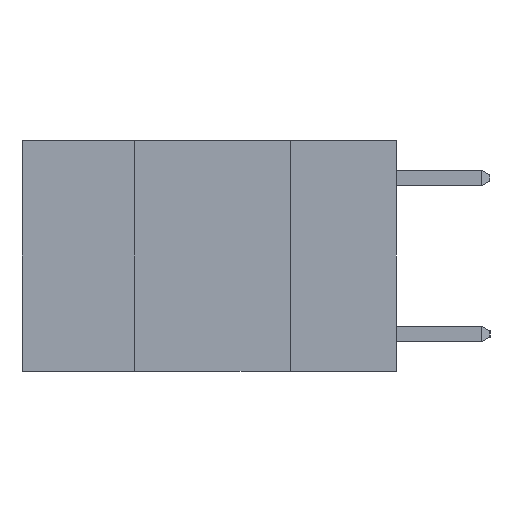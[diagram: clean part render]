
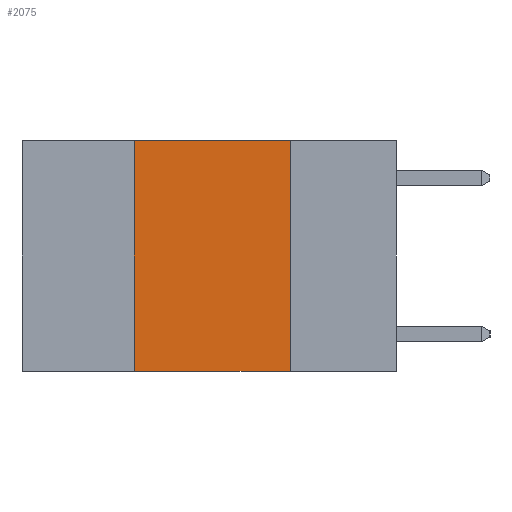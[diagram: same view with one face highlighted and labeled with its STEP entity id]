
A CAD part, left-side view. The second image highlights one B-rep face of the part: STEP entity #2075.
In plain terms, the highlighted planar face has unit normal (-1, 0, 0).
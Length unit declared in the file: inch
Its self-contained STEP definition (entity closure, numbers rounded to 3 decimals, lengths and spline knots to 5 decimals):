
#252 = CARTESIAN_POINT ( 'NONE',  ( 0., 0.6, -0.37 ) ) ;
#378 = EDGE_LOOP ( 'NONE', ( #4096, #4317, #6116, #4519 ) ) ;
#1094 = VECTOR ( 'NONE', #1281, 39.37008 ) ;
#1276 = CARTESIAN_POINT ( 'NONE',  ( 0., 0.42, 0. ) ) ;
#1281 = DIRECTION ( 'NONE',  ( 0., 0., -1. ) ) ;
#1657 = CARTESIAN_POINT ( 'NONE',  ( 0., 0.17, 0. ) ) ;
#2075 = ADVANCED_FACE ( 'NONE', ( #7980 ), #2799, .F. ) ;
#2078 = VECTOR ( 'NONE', #2474, 39.37008 ) ;
#2134 = CARTESIAN_POINT ( 'NONE',  ( 0., 0.17, 0. ) ) ;
#2190 = CARTESIAN_POINT ( 'NONE',  ( 0., 0.6, 0. ) ) ;
#2298 = EDGE_CURVE ( 'NONE', #8697, #3487, #2957, .T. ) ;
#2377 = EDGE_CURVE ( 'NONE', #8697, #4282, #5681, .T. ) ;
#2474 = DIRECTION ( 'NONE',  ( 0., -1., 0. ) ) ;
#2799 = PLANE ( 'NONE',  #4095 ) ;
#2909 = DIRECTION ( 'NONE',  ( 1., 0., 0. ) ) ;
#2939 = LINE ( 'NONE', #1657, #1094 ) ;
#2957 = LINE ( 'NONE', #1276, #8081 ) ;
#2985 = VECTOR ( 'NONE', #7218, 39.37008 ) ;
#3204 = VERTEX_POINT ( 'NONE', #2134 ) ;
#3212 = EDGE_CURVE ( 'NONE', #3204, #4282, #2939, .T. ) ;
#3487 = VERTEX_POINT ( 'NONE', #5888 ) ;
#4095 = AXIS2_PLACEMENT_3D ( 'NONE', #2190, #2909, #4097 ) ;
#4096 = ORIENTED_EDGE ( 'NONE', *, *, #3212, .F. ) ;
#4097 = DIRECTION ( 'NONE',  ( 0., 0., -1. ) ) ;
#4282 = VERTEX_POINT ( 'NONE', #7170 ) ;
#4317 = ORIENTED_EDGE ( 'NONE', *, *, #8198, .F. ) ;
#4519 = ORIENTED_EDGE ( 'NONE', *, *, #2377, .T. ) ;
#5395 = DIRECTION ( 'NONE',  ( 0., 0., 1. ) ) ;
#5681 = LINE ( 'NONE', #252, #2078 ) ;
#5888 = CARTESIAN_POINT ( 'NONE',  ( 0., 0.42, 0. ) ) ;
#6116 = ORIENTED_EDGE ( 'NONE', *, *, #2298, .F. ) ;
#6578 = CARTESIAN_POINT ( 'NONE',  ( 0., 0.6, 0. ) ) ;
#7079 = CARTESIAN_POINT ( 'NONE',  ( 0., 0.42, -0.37 ) ) ;
#7170 = CARTESIAN_POINT ( 'NONE',  ( 0., 0.17, -0.37 ) ) ;
#7218 = DIRECTION ( 'NONE',  ( 0., -1., 0. ) ) ;
#7980 = FACE_OUTER_BOUND ( 'NONE', #378, .T. ) ;
#8081 = VECTOR ( 'NONE', #5395, 39.37008 ) ;
#8198 = EDGE_CURVE ( 'NONE', #3487, #3204, #8326, .T. ) ;
#8326 = LINE ( 'NONE', #6578, #2985 ) ;
#8697 = VERTEX_POINT ( 'NONE', #7079 ) ;
